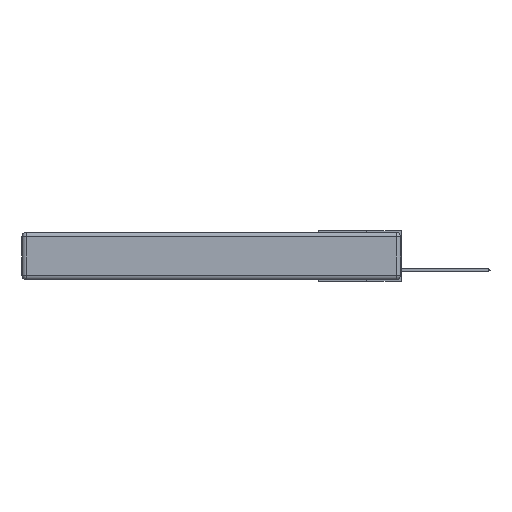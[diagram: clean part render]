
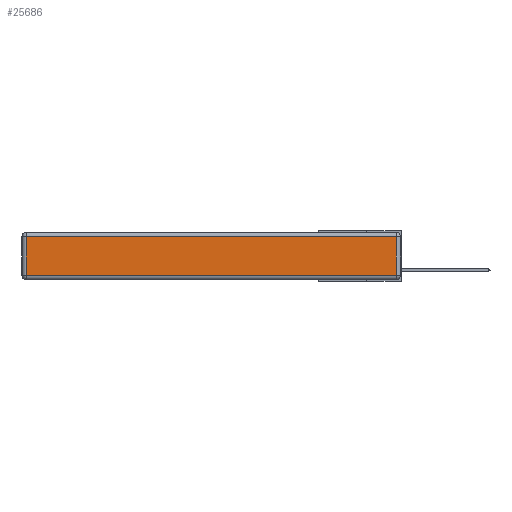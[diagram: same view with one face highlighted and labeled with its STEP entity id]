
A CAD part, left-side view. The second image highlights one B-rep face of the part: STEP entity #25686.
In plain terms, the highlighted planar face has unit normal (-1, 0, 0).
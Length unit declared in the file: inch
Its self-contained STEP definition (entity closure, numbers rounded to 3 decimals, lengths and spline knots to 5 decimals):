
#368 = EDGE_CURVE ( 'NONE', #9718, #23307, #18157, .T. ) ;
#1730 = PLANE ( 'NONE',  #15548 ) ;
#2547 = DIRECTION ( 'NONE',  ( 0., -1., 0. ) ) ;
#3472 = VECTOR ( 'NONE', #21203, 39.37008 ) ;
#3973 = EDGE_CURVE ( 'NONE', #6051, #9718, #9513, .T. ) ;
#4547 = VECTOR ( 'NONE', #11164, 39.37008 ) ;
#5670 = DIRECTION ( 'NONE',  ( 0., 0., 1. ) ) ;
#5736 = EDGE_CURVE ( 'NONE', #9910, #6051, #9093, .T. ) ;
#6051 = VERTEX_POINT ( 'NONE', #16519 ) ;
#6226 = CARTESIAN_POINT ( 'NONE',  ( 0., 0.03, -0.343 ) ) ;
#6635 = ORIENTED_EDGE ( 'NONE', *, *, #5736, .T. ) ;
#8532 = CARTESIAN_POINT ( 'NONE',  ( 0., 0.03, -0.313 ) ) ;
#8889 = FACE_OUTER_BOUND ( 'NONE', #24976, .T. ) ;
#9093 = LINE ( 'NONE', #13079, #3472 ) ;
#9513 = LINE ( 'NONE', #22899, #17047 ) ;
#9718 = VERTEX_POINT ( 'NONE', #8532 ) ;
#9910 = VERTEX_POINT ( 'NONE', #21107 ) ;
#10073 = ORIENTED_EDGE ( 'NONE', *, *, #24675, .T. ) ;
#10436 = DIRECTION ( 'NONE',  ( 0., 0., 1. ) ) ;
#11164 = DIRECTION ( 'NONE',  ( 0., 1., 0. ) ) ;
#12724 = LINE ( 'NONE', #15235, #4547 ) ;
#13079 = CARTESIAN_POINT ( 'NONE',  ( 0., 2.72, -0.343 ) ) ;
#13445 = VECTOR ( 'NONE', #10436, 39.37008 ) ;
#13755 = DIRECTION ( 'NONE',  ( -1., 0., 0. ) ) ;
#15235 = CARTESIAN_POINT ( 'NONE',  ( 0., 2.75, -0.03 ) ) ;
#15548 = AXIS2_PLACEMENT_3D ( 'NONE', #23714, #13755, #5670 ) ;
#15755 = ORIENTED_EDGE ( 'NONE', *, *, #3973, .T. ) ;
#16519 = CARTESIAN_POINT ( 'NONE',  ( 0., 2.72, -0.313 ) ) ;
#17047 = VECTOR ( 'NONE', #2547, 39.37008 ) ;
#18157 = LINE ( 'NONE', #6226, #13445 ) ;
#18306 = ORIENTED_EDGE ( 'NONE', *, *, #368, .T. ) ;
#18986 = CARTESIAN_POINT ( 'NONE',  ( 0., 0.03, -0.03 ) ) ;
#21107 = CARTESIAN_POINT ( 'NONE',  ( 0., 2.72, -0.03 ) ) ;
#21203 = DIRECTION ( 'NONE',  ( 0., 0., -1. ) ) ;
#22899 = CARTESIAN_POINT ( 'NONE',  ( 0., 0., -0.313 ) ) ;
#23307 = VERTEX_POINT ( 'NONE', #18986 ) ;
#23714 = CARTESIAN_POINT ( 'NONE',  ( 0., 0., -0.343 ) ) ;
#24675 = EDGE_CURVE ( 'NONE', #23307, #9910, #12724, .T. ) ;
#24976 = EDGE_LOOP ( 'NONE', ( #15755, #18306, #10073, #6635 ) ) ;
#25686 = ADVANCED_FACE ( 'NONE', ( #8889 ), #1730, .T. ) ;
